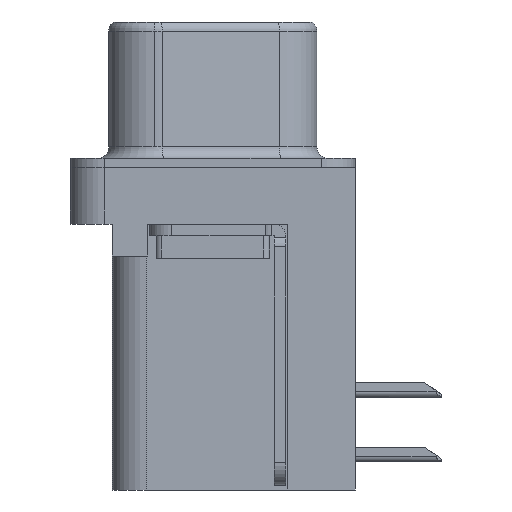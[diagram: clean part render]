
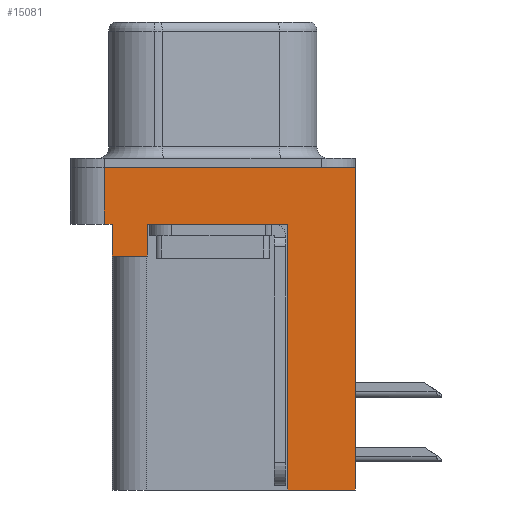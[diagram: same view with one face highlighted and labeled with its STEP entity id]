
A CAD part, left-side view. The second image highlights one B-rep face of the part: STEP entity #15081.
In plain terms, the highlighted planar face has unit normal (-1, 0, 0).
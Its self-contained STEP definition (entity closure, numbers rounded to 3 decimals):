
#170 = VERTEX_POINT ( 'NONE', #8271 ) ;
#192 = CARTESIAN_POINT ( 'NONE',  ( -2.935, 4.425, -3.9 ) ) ;
#303 = ORIENTED_EDGE ( 'NONE', *, *, #7887, .T. ) ;
#942 = EDGE_CURVE ( 'NONE', #18453, #17784, #13461, .T. ) ;
#1011 = VERTEX_POINT ( 'NONE', #1980 ) ;
#1234 = VECTOR ( 'NONE', #11774, 1000. ) ;
#1351 = ORIENTED_EDGE ( 'NONE', *, *, #10392, .F. ) ;
#1755 = VECTOR ( 'NONE', #15503, 1000. ) ;
#1980 = CARTESIAN_POINT ( 'NONE',  ( -2.935, 2.895, -2.5 ) ) ;
#2742 = EDGE_CURVE ( 'NONE', #5687, #1011, #4217, .T. ) ;
#2826 = VECTOR ( 'NONE', #10842, 1000. ) ;
#2878 = VERTEX_POINT ( 'NONE', #11740 ) ;
#3007 = VECTOR ( 'NONE', #12547, 1000. ) ;
#3219 = VERTEX_POINT ( 'NONE', #8246 ) ;
#3282 = VECTOR ( 'NONE', #15884, 1000. ) ;
#3557 = EDGE_CURVE ( 'NONE', #14697, #170, #8313, .T. ) ;
#3582 = DIRECTION ( 'NONE',  ( 0., 0., 1. ) ) ;
#3788 = CARTESIAN_POINT ( 'NONE',  ( -2.935, -6.275, -14.2 ) ) ;
#3938 = CARTESIAN_POINT ( 'NONE',  ( -2.935, 2.895, -3.9 ) ) ;
#4199 = VECTOR ( 'NONE', #6776, 1000. ) ;
#4217 = LINE ( 'NONE', #3938, #4199 ) ;
#4226 = VECTOR ( 'NONE', #15251, 1000. ) ;
#4544 = VECTOR ( 'NONE', #8426, 1000. ) ;
#5212 = CARTESIAN_POINT ( 'NONE',  ( -2.935, -3.295, -14.2 ) ) ;
#5557 = EDGE_CURVE ( 'NONE', #5687, #14697, #15648, .T. ) ;
#5687 = VERTEX_POINT ( 'NONE', #7473 ) ;
#5763 = EDGE_LOOP ( 'NONE', ( #1351, #8115, #303, #6171, #18033, #15600, #9798, #10150, #6018, #14844 ) ) ;
#6018 = ORIENTED_EDGE ( 'NONE', *, *, #11184, .F. ) ;
#6171 = ORIENTED_EDGE ( 'NONE', *, *, #3557, .F. ) ;
#6776 = DIRECTION ( 'NONE',  ( 0., 0., 1. ) ) ;
#6982 = LINE ( 'NONE', #12984, #3282 ) ;
#7064 = LINE ( 'NONE', #15692, #1755 ) ;
#7473 = CARTESIAN_POINT ( 'NONE',  ( -2.935, 2.895, -3.9 ) ) ;
#7887 = EDGE_CURVE ( 'NONE', #2878, #170, #7064, .T. ) ;
#8115 = ORIENTED_EDGE ( 'NONE', *, *, #12147, .F. ) ;
#8206 = LINE ( 'NONE', #12350, #17748 ) ;
#8246 = CARTESIAN_POINT ( 'NONE',  ( -2.935, -3.295, -2.5 ) ) ;
#8271 = CARTESIAN_POINT ( 'NONE',  ( -2.935, 4.425, -2.5 ) ) ;
#8313 = LINE ( 'NONE', #16670, #4226 ) ;
#8315 = CARTESIAN_POINT ( 'NONE',  ( -2.935, -3.295, -14.2 ) ) ;
#8426 = DIRECTION ( 'NONE',  ( 0., 1., 0. ) ) ;
#8594 = CARTESIAN_POINT ( 'NONE',  ( -2.935, -6.275, -2.5 ) ) ;
#9327 = CARTESIAN_POINT ( 'NONE',  ( -2.935, -6.275, -2.5 ) ) ;
#9798 = ORIENTED_EDGE ( 'NONE', *, *, #9909, .T. ) ;
#9909 = EDGE_CURVE ( 'NONE', #1011, #3219, #10097, .T. ) ;
#10097 = LINE ( 'NONE', #8594, #10804 ) ;
#10150 = ORIENTED_EDGE ( 'NONE', *, *, #12460, .F. ) ;
#10392 = EDGE_CURVE ( 'NONE', #13714, #17784, #6982, .T. ) ;
#10551 = LINE ( 'NONE', #16259, #1234 ) ;
#10804 = VECTOR ( 'NONE', #12735, 1000. ) ;
#10842 = DIRECTION ( 'NONE',  ( 0., 0., 1. ) ) ;
#11064 = DIRECTION ( 'NONE',  ( 0., 0., 1. ) ) ;
#11184 = EDGE_CURVE ( 'NONE', #18453, #18419, #13763, .T. ) ;
#11659 = CARTESIAN_POINT ( 'NONE',  ( -2.935, -6.275, 0. ) ) ;
#11740 = CARTESIAN_POINT ( 'NONE',  ( -2.935, 4.775, -2.5 ) ) ;
#11774 = DIRECTION ( 'NONE',  ( 0., 0., 1. ) ) ;
#12147 = EDGE_CURVE ( 'NONE', #2878, #13714, #8206, .T. ) ;
#12350 = CARTESIAN_POINT ( 'NONE',  ( -2.935, 4.775, -2.5 ) ) ;
#12460 = EDGE_CURVE ( 'NONE', #18419, #3219, #10551, .T. ) ;
#12547 = DIRECTION ( 'NONE',  ( 0., 1., 0. ) ) ;
#12735 = DIRECTION ( 'NONE',  ( 0., -1., 0. ) ) ;
#12984 = CARTESIAN_POINT ( 'NONE',  ( -2.935, -6.275, 0. ) ) ;
#13461 = LINE ( 'NONE', #9327, #2826 ) ;
#13714 = VERTEX_POINT ( 'NONE', #16766 ) ;
#13763 = LINE ( 'NONE', #8315, #3007 ) ;
#14056 = FACE_OUTER_BOUND ( 'NONE', #5763, .T. ) ;
#14252 = DIRECTION ( 'NONE',  ( -1., 0., 0. ) ) ;
#14697 = VERTEX_POINT ( 'NONE', #15397 ) ;
#14807 = AXIS2_PLACEMENT_3D ( 'NONE', #15467, #14252, #11064 ) ;
#14844 = ORIENTED_EDGE ( 'NONE', *, *, #942, .T. ) ;
#15081 = ADVANCED_FACE ( 'NONE', ( #14056 ), #18270, .T. ) ;
#15251 = DIRECTION ( 'NONE',  ( 0., 0., 1. ) ) ;
#15397 = CARTESIAN_POINT ( 'NONE',  ( -2.935, 4.425, -3.9 ) ) ;
#15467 = CARTESIAN_POINT ( 'NONE',  ( -2.935, -6.275, -2.5 ) ) ;
#15503 = DIRECTION ( 'NONE',  ( 0., -1., 0. ) ) ;
#15600 = ORIENTED_EDGE ( 'NONE', *, *, #2742, .T. ) ;
#15648 = LINE ( 'NONE', #192, #4544 ) ;
#15692 = CARTESIAN_POINT ( 'NONE',  ( -2.935, -6.275, -2.5 ) ) ;
#15884 = DIRECTION ( 'NONE',  ( 0., -1., 0. ) ) ;
#16259 = CARTESIAN_POINT ( 'NONE',  ( -2.935, -3.295, -14.2 ) ) ;
#16670 = CARTESIAN_POINT ( 'NONE',  ( -2.935, 4.425, -3.9 ) ) ;
#16766 = CARTESIAN_POINT ( 'NONE',  ( -2.935, 4.775, 0. ) ) ;
#17748 = VECTOR ( 'NONE', #3582, 1000. ) ;
#17784 = VERTEX_POINT ( 'NONE', #11659 ) ;
#18033 = ORIENTED_EDGE ( 'NONE', *, *, #5557, .F. ) ;
#18270 = PLANE ( 'NONE',  #14807 ) ;
#18419 = VERTEX_POINT ( 'NONE', #5212 ) ;
#18453 = VERTEX_POINT ( 'NONE', #3788 ) ;
